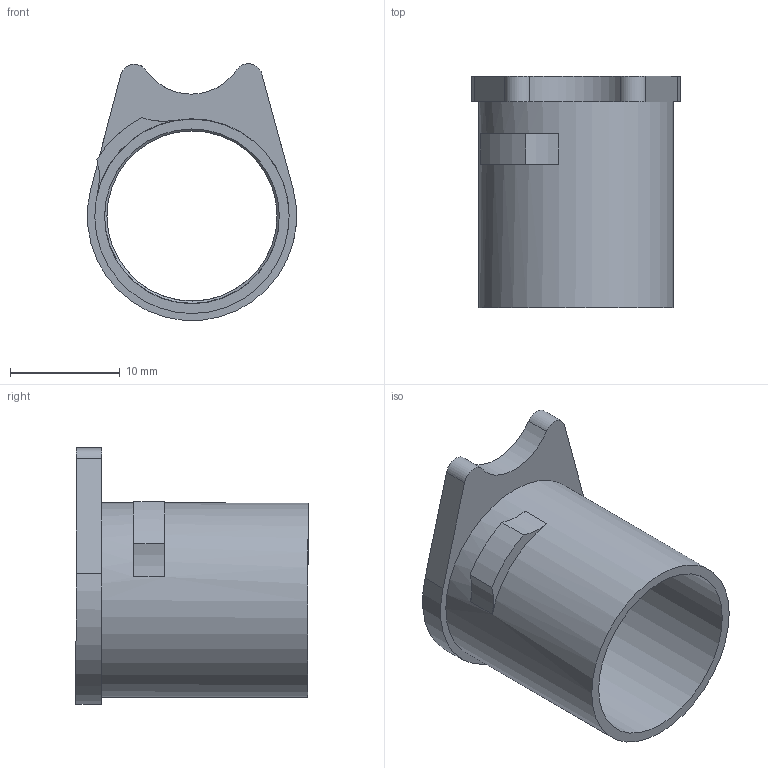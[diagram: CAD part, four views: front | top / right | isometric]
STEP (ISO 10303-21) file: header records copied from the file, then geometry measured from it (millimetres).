
FILE_DESCRIPTION(('FreeCAD Model'),'2;1');
FILE_NAME('M1911 Barrel Bushing.step', '2017-11-15T18:25:08',('Author'),(''), 'Open CASCADE STEP processor 6.8','FreeCAD','Unknown');
FILE_SCHEMA(('AUTOMOTIVE_DESIGN_CC2 { 1 2 10303 214 -1 1 5 4 }'));
Length unit declared in the file: millimetre
Products named in the file (1): 1911_Barrel_Bushing
Bounding box: 18.99 x 21.12 x 23.34 mm (x, y, z)
Volume: 1309.7 mm3; surface area: 2583.2 mm2
Topology: 1 solids, 1 shells, 20 faces, 50 edges, 35 vertices
Faces by surface type: cylinder 11, plane 8, cone 1
Full cylindrical faces by diameter (mm): 15.476 x1, 15.494 x1, 15.894 x1, 17.678 x1
Entity records: 2584 total; most frequent: CARTESIAN_POINT 1634, DIRECTION 156, ORIENTED_EDGE 100, PCURVE 100, DEFINITIONAL_REPRESENTATION 100, B_SPLINE_CURVE_WITH_KNOTS 57, AXIS2_PLACEMENT_3D 52, EDGE_CURVE 50
